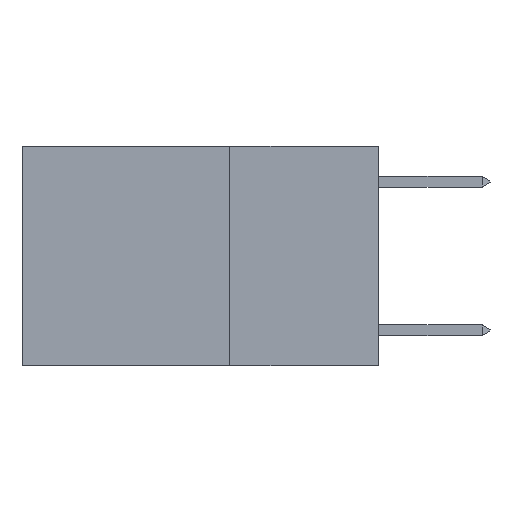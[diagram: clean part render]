
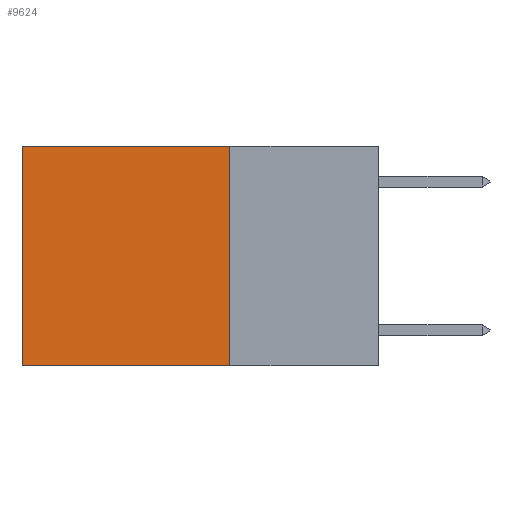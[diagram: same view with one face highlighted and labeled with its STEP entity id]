
A CAD part, left-side view. The second image highlights one B-rep face of the part: STEP entity #9624.
In plain terms, the highlighted planar face has unit normal (-1, 0, 0).
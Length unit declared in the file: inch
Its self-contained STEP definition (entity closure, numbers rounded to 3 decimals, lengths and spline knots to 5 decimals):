
#66 = EDGE_CURVE ( 'NONE', #354, #6078, #9714, .T. ) ;
#354 = VERTEX_POINT ( 'NONE', #6761 ) ;
#420 = VERTEX_POINT ( 'NONE', #3781 ) ;
#496 = DIRECTION ( 'NONE',  ( 0., 1., 0. ) ) ;
#1811 = DIRECTION ( 'NONE',  ( 0., 0., -1. ) ) ;
#2363 = VECTOR ( 'NONE', #6817, 39.37008 ) ;
#3317 = ORIENTED_EDGE ( 'NONE', *, *, #5980, .F. ) ;
#3781 = CARTESIAN_POINT ( 'NONE',  ( 0.2625, 0.25, 0. ) ) ;
#3985 = AXIS2_PLACEMENT_3D ( 'NONE', #6502, #9444, #1811 ) ;
#4214 = VECTOR ( 'NONE', #5322, 39.37008 ) ;
#4530 = EDGE_LOOP ( 'NONE', ( #5270, #7486, #3317, #12049 ) ) ;
#5270 = ORIENTED_EDGE ( 'NONE', *, *, #12011, .T. ) ;
#5322 = DIRECTION ( 'NONE',  ( 0., 0., -1. ) ) ;
#5394 = CARTESIAN_POINT ( 'NONE',  ( 0.2625, 0.6, -0.37 ) ) ;
#5716 = FACE_OUTER_BOUND ( 'NONE', #4530, .T. ) ;
#5782 = LINE ( 'NONE', #7566, #2363 ) ;
#5980 = EDGE_CURVE ( 'NONE', #420, #354, #8117, .T. ) ;
#6078 = VERTEX_POINT ( 'NONE', #5394 ) ;
#6379 = PLANE ( 'NONE',  #3985 ) ;
#6502 = CARTESIAN_POINT ( 'NONE',  ( 0.2625, 0.25, 0. ) ) ;
#6761 = CARTESIAN_POINT ( 'NONE',  ( 0.2625, 0.25, -0.37 ) ) ;
#6817 = DIRECTION ( 'NONE',  ( 0., 0., -1. ) ) ;
#7486 = ORIENTED_EDGE ( 'NONE', *, *, #66, .F. ) ;
#7566 = CARTESIAN_POINT ( 'NONE',  ( 0.2625, 0.6, 0. ) ) ;
#7741 = VERTEX_POINT ( 'NONE', #10015 ) ;
#8117 = LINE ( 'NONE', #9849, #4214 ) ;
#8549 = CARTESIAN_POINT ( 'NONE',  ( 0.2625, 0.25, -0.37 ) ) ;
#8782 = DIRECTION ( 'NONE',  ( 0., 1., 0. ) ) ;
#8820 = CARTESIAN_POINT ( 'NONE',  ( 0.2625, 0.25, 0. ) ) ;
#8883 = LINE ( 'NONE', #8820, #10236 ) ;
#9444 = DIRECTION ( 'NONE',  ( 1., 0., 0. ) ) ;
#9624 = ADVANCED_FACE ( 'NONE', ( #5716 ), #6379, .F. ) ;
#9714 = LINE ( 'NONE', #8549, #11963 ) ;
#9849 = CARTESIAN_POINT ( 'NONE',  ( 0.2625, 0.25, 0. ) ) ;
#10015 = CARTESIAN_POINT ( 'NONE',  ( 0.2625, 0.6, 0. ) ) ;
#10236 = VECTOR ( 'NONE', #496, 39.37008 ) ;
#10850 = EDGE_CURVE ( 'NONE', #420, #7741, #8883, .T. ) ;
#11963 = VECTOR ( 'NONE', #8782, 39.37008 ) ;
#12011 = EDGE_CURVE ( 'NONE', #7741, #6078, #5782, .T. ) ;
#12049 = ORIENTED_EDGE ( 'NONE', *, *, #10850, .T. ) ;
